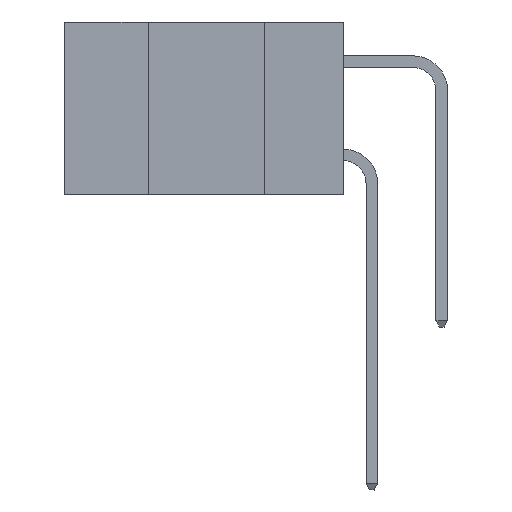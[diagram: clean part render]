
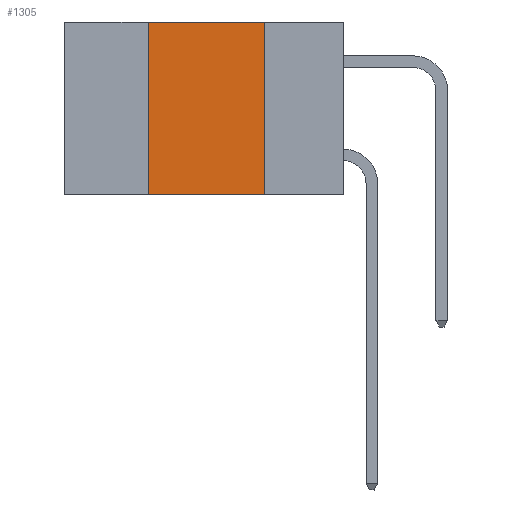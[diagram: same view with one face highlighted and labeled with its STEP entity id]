
A CAD part, left-side view. The second image highlights one B-rep face of the part: STEP entity #1305.
In plain terms, the highlighted planar face has unit normal (-1, 0, 0).
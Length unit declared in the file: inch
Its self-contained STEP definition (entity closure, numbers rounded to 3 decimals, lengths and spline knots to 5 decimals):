
#678 = CARTESIAN_POINT ( 'NONE',  ( 0., 0.6, 0. ) ) ;
#1093 = EDGE_CURVE ( 'NONE', #11199, #2296, #8726, .T. ) ;
#1155 = DIRECTION ( 'NONE',  ( 0., 0., -1. ) ) ;
#1305 = ADVANCED_FACE ( 'NONE', ( #15895 ), #4365, .F. ) ;
#1727 = CARTESIAN_POINT ( 'NONE',  ( 0., 0.17, -0.37 ) ) ;
#1868 = CARTESIAN_POINT ( 'NONE',  ( 0., 0.42, -0.37 ) ) ;
#2296 = VERTEX_POINT ( 'NONE', #1727 ) ;
#2812 = ORIENTED_EDGE ( 'NONE', *, *, #5568, .F. ) ;
#3092 = ORIENTED_EDGE ( 'NONE', *, *, #4882, .F. ) ;
#3334 = EDGE_CURVE ( 'NONE', #11199, #13538, #14226, .T. ) ;
#3956 = ORIENTED_EDGE ( 'NONE', *, *, #1093, .T. ) ;
#4112 = DIRECTION ( 'NONE',  ( 1., 0., 0. ) ) ;
#4322 = VECTOR ( 'NONE', #1155, 39.37008 ) ;
#4365 = PLANE ( 'NONE',  #9907 ) ;
#4724 = ORIENTED_EDGE ( 'NONE', *, *, #3334, .F. ) ;
#4882 = EDGE_CURVE ( 'NONE', #13538, #8606, #12226, .T. ) ;
#5568 = EDGE_CURVE ( 'NONE', #8606, #2296, #13153, .T. ) ;
#6351 = VECTOR ( 'NONE', #15520, 39.37008 ) ;
#6774 = DIRECTION ( 'NONE',  ( 0., 0., -1. ) ) ;
#8442 = VECTOR ( 'NONE', #10788, 39.37008 ) ;
#8606 = VERTEX_POINT ( 'NONE', #15701 ) ;
#8610 = VECTOR ( 'NONE', #15573, 39.37008 ) ;
#8726 = LINE ( 'NONE', #11350, #6351 ) ;
#9907 = AXIS2_PLACEMENT_3D ( 'NONE', #13282, #4112, #6774 ) ;
#10205 = CARTESIAN_POINT ( 'NONE',  ( 0., 0.42, -0.37 ) ) ;
#10788 = DIRECTION ( 'NONE',  ( 0., -1., 0. ) ) ;
#11199 = VERTEX_POINT ( 'NONE', #1868 ) ;
#11350 = CARTESIAN_POINT ( 'NONE',  ( 0., 0.6, -0.37 ) ) ;
#12226 = LINE ( 'NONE', #678, #8442 ) ;
#12692 = CARTESIAN_POINT ( 'NONE',  ( 0., 0.17, -0.37 ) ) ;
#12765 = CARTESIAN_POINT ( 'NONE',  ( 0., 0.42, 0. ) ) ;
#13153 = LINE ( 'NONE', #12692, #4322 ) ;
#13282 = CARTESIAN_POINT ( 'NONE',  ( 0., 0.6, 0. ) ) ;
#13538 = VERTEX_POINT ( 'NONE', #12765 ) ;
#14226 = LINE ( 'NONE', #10205, #8610 ) ;
#15520 = DIRECTION ( 'NONE',  ( 0., -1., 0. ) ) ;
#15573 = DIRECTION ( 'NONE',  ( 0., 0., 1. ) ) ;
#15701 = CARTESIAN_POINT ( 'NONE',  ( 0., 0.17, 0. ) ) ;
#15895 = FACE_OUTER_BOUND ( 'NONE', #16585, .T. ) ;
#16585 = EDGE_LOOP ( 'NONE', ( #2812, #3092, #4724, #3956 ) ) ;
